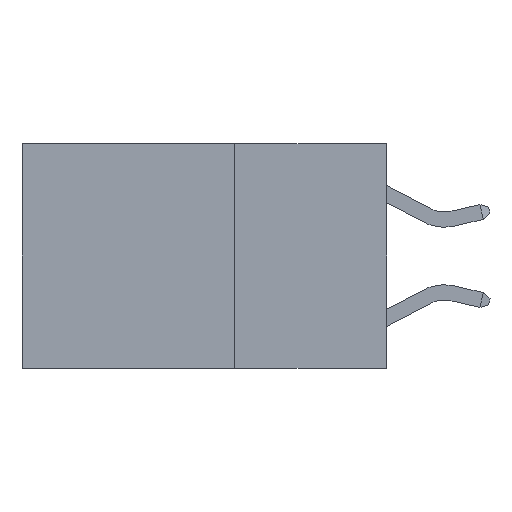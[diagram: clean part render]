
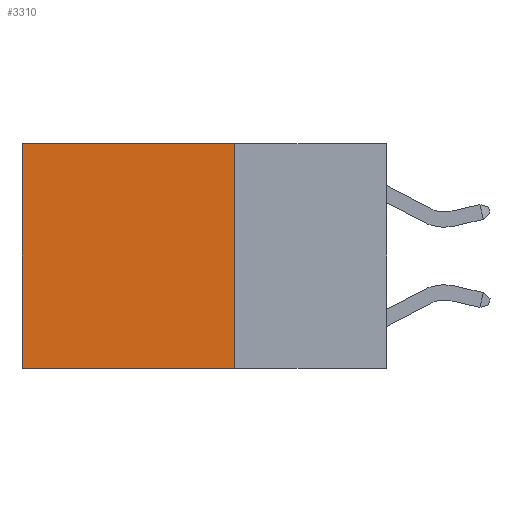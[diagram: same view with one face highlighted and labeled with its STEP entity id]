
A CAD part, left-side view. The second image highlights one B-rep face of the part: STEP entity #3310.
In plain terms, the highlighted planar face has unit normal (-1, 0, 0).
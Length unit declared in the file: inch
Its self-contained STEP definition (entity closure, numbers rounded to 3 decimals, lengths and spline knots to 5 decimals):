
#176 = EDGE_LOOP ( 'NONE', ( #10314, #1560, #1846, #4348 ) ) ;
#352 = VERTEX_POINT ( 'NONE', #11230 ) ;
#858 = EDGE_CURVE ( 'NONE', #4748, #6474, #10667, .T. ) ;
#885 = CARTESIAN_POINT ( 'NONE',  ( 0.2625, 0.25, 0. ) ) ;
#1560 = ORIENTED_EDGE ( 'NONE', *, *, #3950, .F. ) ;
#1589 = EDGE_CURVE ( 'NONE', #352, #1687, #10426, .T. ) ;
#1687 = VERTEX_POINT ( 'NONE', #10342 ) ;
#1739 = LINE ( 'NONE', #8500, #8564 ) ;
#1846 = ORIENTED_EDGE ( 'NONE', *, *, #858, .F. ) ;
#2399 = DIRECTION ( 'NONE',  ( 0., 0., -1. ) ) ;
#2936 = VECTOR ( 'NONE', #8049, 39.37008 ) ;
#3169 = CARTESIAN_POINT ( 'NONE',  ( 0.2625, 0.25, 0. ) ) ;
#3183 = CARTESIAN_POINT ( 'NONE',  ( 0.2625, 0.25, 0. ) ) ;
#3310 = ADVANCED_FACE ( 'NONE', ( #7431 ), #4118, .F. ) ;
#3583 = VECTOR ( 'NONE', #8240, 39.37008 ) ;
#3788 = CARTESIAN_POINT ( 'NONE',  ( 0.2625, 0.25, -0.37 ) ) ;
#3950 = EDGE_CURVE ( 'NONE', #6474, #1687, #7677, .T. ) ;
#4118 = PLANE ( 'NONE',  #10775 ) ;
#4348 = ORIENTED_EDGE ( 'NONE', *, *, #4786, .T. ) ;
#4748 = VERTEX_POINT ( 'NONE', #3169 ) ;
#4786 = EDGE_CURVE ( 'NONE', #4748, #352, #1739, .T. ) ;
#5047 = DIRECTION ( 'NONE',  ( 1., 0., 0. ) ) ;
#6474 = VERTEX_POINT ( 'NONE', #3788 ) ;
#7162 = CARTESIAN_POINT ( 'NONE',  ( 0.2625, 0.25, -0.37 ) ) ;
#7431 = FACE_OUTER_BOUND ( 'NONE', #176, .T. ) ;
#7677 = LINE ( 'NONE', #7162, #2936 ) ;
#8049 = DIRECTION ( 'NONE',  ( 0., 1., 0. ) ) ;
#8240 = DIRECTION ( 'NONE',  ( 0., 0., -1. ) ) ;
#8500 = CARTESIAN_POINT ( 'NONE',  ( 0.2625, 0.25, 0. ) ) ;
#8564 = VECTOR ( 'NONE', #9316, 39.37008 ) ;
#9316 = DIRECTION ( 'NONE',  ( 0., 1., 0. ) ) ;
#10170 = VECTOR ( 'NONE', #2399, 39.37008 ) ;
#10196 = CARTESIAN_POINT ( 'NONE',  ( 0.2625, 0.6, 0. ) ) ;
#10314 = ORIENTED_EDGE ( 'NONE', *, *, #1589, .T. ) ;
#10342 = CARTESIAN_POINT ( 'NONE',  ( 0.2625, 0.6, -0.37 ) ) ;
#10426 = LINE ( 'NONE', #10196, #10170 ) ;
#10667 = LINE ( 'NONE', #885, #3583 ) ;
#10775 = AXIS2_PLACEMENT_3D ( 'NONE', #3183, #5047, #10887 ) ;
#10887 = DIRECTION ( 'NONE',  ( 0., 0., -1. ) ) ;
#11230 = CARTESIAN_POINT ( 'NONE',  ( 0.2625, 0.6, 0. ) ) ;
